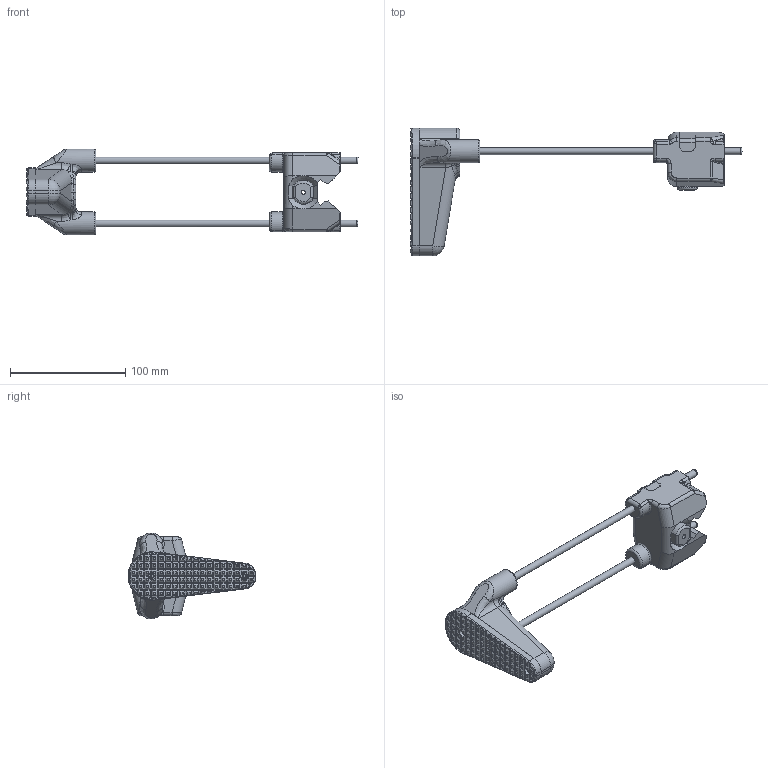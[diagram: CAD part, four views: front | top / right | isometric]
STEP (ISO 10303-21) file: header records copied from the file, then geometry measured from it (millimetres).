
FILE_DESCRIPTION(/* description */ (''),/* implementation_level */ '2;1');
FILE_NAME(/* name */ 'mp5a3.stp',/* time_stamp */ '2021-01-23T20:20:25+02:00',/* author */ (''),/* organization */ (''),/* preprocessor_version */ 'ST-DEVELOPER v15.2',/* originating_system */ 'Autodesk Translator Framework v2.0.0.5431',/* authorisation */ '');
FILE_SCHEMA (('AUTOMOTIVE_DESIGN { 1 0 10303 214 3 1 1 }'));
Length unit declared in the file: centimetre
Products named in the file (1): (Unsaved)
Bounding box: 288.15 x 111.08 x 74.61 mm (x, y, z)
Volume: 255182.8 mm3; surface area: 73112.9 mm2
Topology: 7 solids, 7 shells, 1057 faces, 2527 edges, 1486 vertices
Faces by surface type: plane 612, bspline 306, cylinder 95, torus 21, cone 13, sphere 10
Full cylindrical faces by diameter (mm): 2.5 x2, 3.5 x1, 3.7 x2, 4 x2, 6 x6, 8 x1, 10 x1, 13 x1, 20 x3, 25.45 x1
Entity records: 34248 total; most frequent: CARTESIAN_POINT 11132, ORIENTED_EDGE 4948, DIRECTION 4589, EDGE_CURVE 2474, AXIS2_PLACEMENT_3D 1588, VERTEX_POINT 1471, LINE 1413, VECTOR 1413
